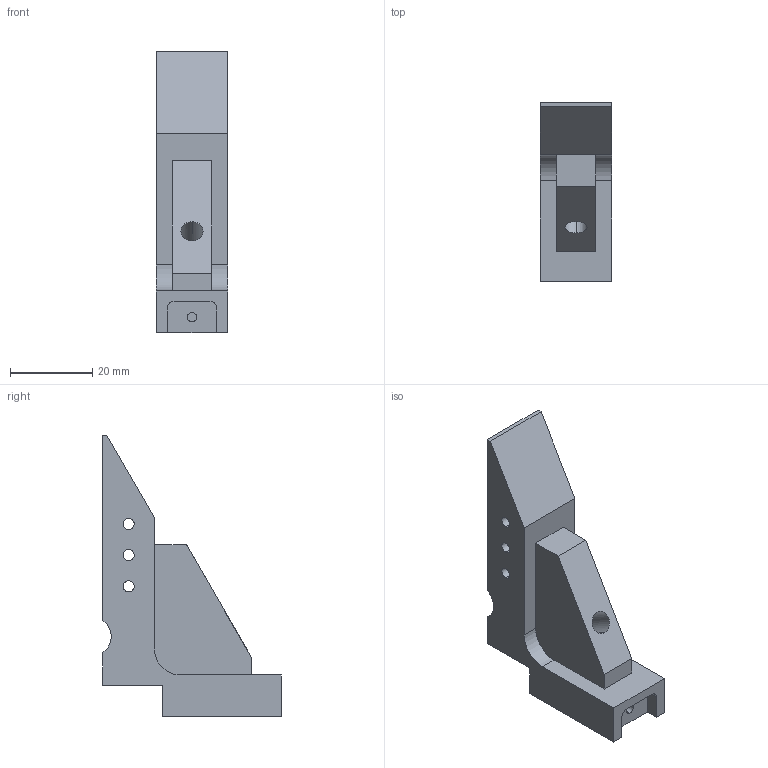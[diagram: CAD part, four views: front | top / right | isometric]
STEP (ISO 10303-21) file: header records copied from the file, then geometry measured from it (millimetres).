
FILE_DESCRIPTION (( 'STEP AP214' ), '1' );
FILE_NAME ('Original_Grip_Part.step', '2015-06-12T14:16:54', ( '' ), ( '' ), 'SwSTEP 2.0', 'SolidWorks 2015', '' );
FILE_SCHEMA (( 'AUTOMOTIVE_DESIGN' ));
Length unit declared in the file: inch
Products named in the file (1): Original_Grip_Part
Bounding box: 17.53 x 43.56 x 68.58 mm (x, y, z)
Volume: 18501 mm3; surface area: 8021.1 mm2
Topology: 1 solids, 1 shells, 50 faces, 135 edges, 90 vertices
Faces by surface type: plane 28, cylinder 22
Entity records: 1639 total; most frequent: CARTESIAN_POINT 288, DIRECTION 275, ORIENTED_EDGE 270, EDGE_CURVE 135, AXIS2_PLACEMENT_3D 93, VERTEX_POINT 90, VECTOR 89, LINE 89
